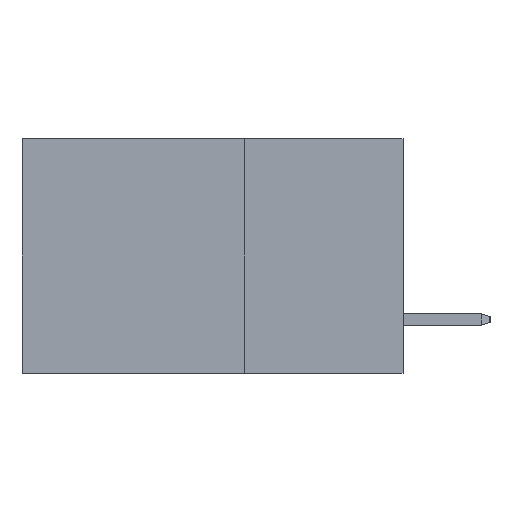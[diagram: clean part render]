
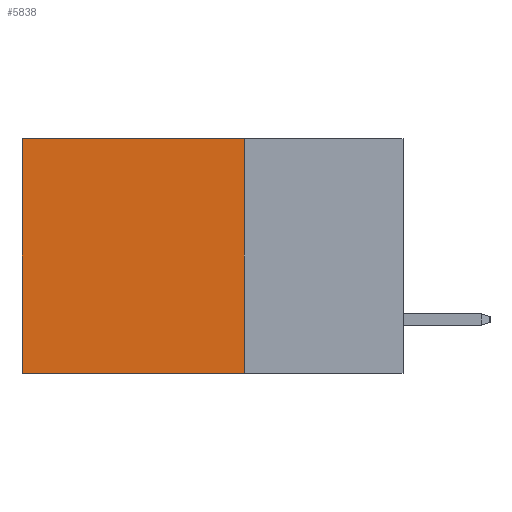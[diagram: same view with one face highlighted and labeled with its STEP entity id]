
A CAD part, left-side view. The second image highlights one B-rep face of the part: STEP entity #5838.
In plain terms, the highlighted planar face has unit normal (-1, 0, 0).
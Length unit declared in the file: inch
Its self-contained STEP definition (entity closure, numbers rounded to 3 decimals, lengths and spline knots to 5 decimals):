
#130 = CARTESIAN_POINT ( 'NONE',  ( 0.2875, 0.25, 0. ) ) ;
#269 = CARTESIAN_POINT ( 'NONE',  ( 0.2875, 0.25, -0.37 ) ) ;
#444 = DIRECTION ( 'NONE',  ( 0., 1., 0. ) ) ;
#688 = EDGE_CURVE ( 'NONE', #3277, #3530, #6491, .T. ) ;
#886 = DIRECTION ( 'NONE',  ( 0., 0., -1. ) ) ;
#2378 = VECTOR ( 'NONE', #9997, 39.37008 ) ;
#2380 = ORIENTED_EDGE ( 'NONE', *, *, #688, .F. ) ;
#2829 = VECTOR ( 'NONE', #8178, 39.37008 ) ;
#2960 = EDGE_CURVE ( 'NONE', #10609, #3706, #7254, .T. ) ;
#3169 = ORIENTED_EDGE ( 'NONE', *, *, #7591, .F. ) ;
#3197 = CARTESIAN_POINT ( 'NONE',  ( 0.2875, 0.25, 0. ) ) ;
#3277 = VERTEX_POINT ( 'NONE', #8640 ) ;
#3333 = VECTOR ( 'NONE', #4009, 39.37008 ) ;
#3453 = LINE ( 'NONE', #6740, #2378 ) ;
#3530 = VERTEX_POINT ( 'NONE', #269 ) ;
#3706 = VERTEX_POINT ( 'NONE', #10162 ) ;
#3996 = EDGE_LOOP ( 'NONE', ( #8808, #3169, #2380, #7425 ) ) ;
#4009 = DIRECTION ( 'NONE',  ( 0., 0., -1. ) ) ;
#5109 = DIRECTION ( 'NONE',  ( 1., 0., 0. ) ) ;
#5369 = CARTESIAN_POINT ( 'NONE',  ( 0.2875, 0.25, -0.37 ) ) ;
#5749 = CARTESIAN_POINT ( 'NONE',  ( 0.2875, 0.6, 0. ) ) ;
#5838 = ADVANCED_FACE ( 'NONE', ( #7572 ), #6662, .F. ) ;
#6193 = AXIS2_PLACEMENT_3D ( 'NONE', #130, #5109, #886 ) ;
#6491 = LINE ( 'NONE', #3197, #3333 ) ;
#6662 = PLANE ( 'NONE',  #6193 ) ;
#6740 = CARTESIAN_POINT ( 'NONE',  ( 0.2875, 0.25, 0. ) ) ;
#6908 = EDGE_CURVE ( 'NONE', #3277, #10609, #3453, .T. ) ;
#7030 = LINE ( 'NONE', #5369, #9408 ) ;
#7254 = LINE ( 'NONE', #5749, #2829 ) ;
#7425 = ORIENTED_EDGE ( 'NONE', *, *, #6908, .T. ) ;
#7572 = FACE_OUTER_BOUND ( 'NONE', #3996, .T. ) ;
#7591 = EDGE_CURVE ( 'NONE', #3530, #3706, #7030, .T. ) ;
#8178 = DIRECTION ( 'NONE',  ( 0., 0., -1. ) ) ;
#8640 = CARTESIAN_POINT ( 'NONE',  ( 0.2875, 0.25, 0. ) ) ;
#8808 = ORIENTED_EDGE ( 'NONE', *, *, #2960, .T. ) ;
#9408 = VECTOR ( 'NONE', #444, 39.37008 ) ;
#9601 = CARTESIAN_POINT ( 'NONE',  ( 0.2875, 0.6, 0. ) ) ;
#9997 = DIRECTION ( 'NONE',  ( 0., 1., 0. ) ) ;
#10162 = CARTESIAN_POINT ( 'NONE',  ( 0.2875, 0.6, -0.37 ) ) ;
#10609 = VERTEX_POINT ( 'NONE', #9601 ) ;
